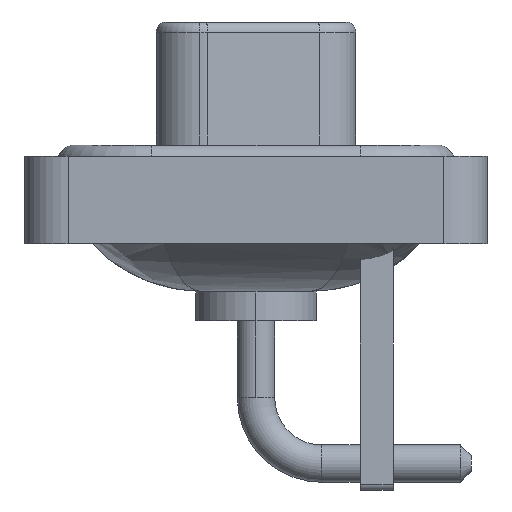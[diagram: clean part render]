
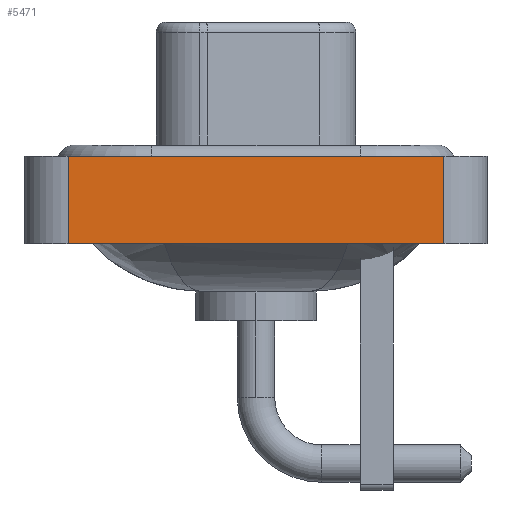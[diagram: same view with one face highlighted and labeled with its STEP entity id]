
A CAD part, left-side view. The second image highlights one B-rep face of the part: STEP entity #5471.
In plain terms, the highlighted planar face has unit normal (-1, 0, 0).
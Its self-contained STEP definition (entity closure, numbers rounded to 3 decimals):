
#958 = VERTEX_POINT ( 'NONE', #18567 ) ;
#1187 = CARTESIAN_POINT ( 'NONE',  ( -7.35, -8.55, 0.4 ) ) ;
#1277 = CARTESIAN_POINT ( 'NONE',  ( -7.35, -8.55, -3.6 ) ) ;
#1954 = CARTESIAN_POINT ( 'NONE',  ( -7.35, -8.55, -3.6 ) ) ;
#2816 = CARTESIAN_POINT ( 'NONE',  ( -7.35, -8.55, -3.6 ) ) ;
#2910 = DIRECTION ( 'NONE',  ( 0., 0., 1. ) ) ;
#4432 = VECTOR ( 'NONE', #15652, 1000. ) ;
#4685 = VECTOR ( 'NONE', #16803, 1000. ) ;
#4875 = EDGE_CURVE ( 'NONE', #958, #12931, #18037, .T. ) ;
#5471 = ADVANCED_FACE ( 'NONE', ( #10415 ), #8712, .T. ) ;
#5986 = ORIENTED_EDGE ( 'NONE', *, *, #4875, .F. ) ;
#6554 = CARTESIAN_POINT ( 'NONE',  ( -7.35, 8.55, 0.4 ) ) ;
#6995 = EDGE_CURVE ( 'NONE', #958, #9778, #15085, .T. ) ;
#7339 = LINE ( 'NONE', #11625, #9507 ) ;
#8279 = AXIS2_PLACEMENT_3D ( 'NONE', #2816, #11577, #2910 ) ;
#8712 = PLANE ( 'NONE',  #8279 ) ;
#9507 = VECTOR ( 'NONE', #13154, 1000. ) ;
#9778 = VERTEX_POINT ( 'NONE', #1277 ) ;
#10415 = FACE_OUTER_BOUND ( 'NONE', #10858, .T. ) ;
#10858 = EDGE_LOOP ( 'NONE', ( #15896, #11590, #5986, #11486 ) ) ;
#11139 = CARTESIAN_POINT ( 'NONE',  ( -7.35, -8.55, 0.4 ) ) ;
#11486 = ORIENTED_EDGE ( 'NONE', *, *, #6995, .T. ) ;
#11577 = DIRECTION ( 'NONE',  ( -1., 0., 0. ) ) ;
#11590 = ORIENTED_EDGE ( 'NONE', *, *, #18526, .F. ) ;
#11625 = CARTESIAN_POINT ( 'NONE',  ( -7.35, -8.55, -3.6 ) ) ;
#12048 = DIRECTION ( 'NONE',  ( 0., 0., 1. ) ) ;
#12931 = VERTEX_POINT ( 'NONE', #6554 ) ;
#13154 = DIRECTION ( 'NONE',  ( 0., 0., 1. ) ) ;
#13719 = EDGE_CURVE ( 'NONE', #9778, #16775, #7339, .T. ) ;
#15085 = LINE ( 'NONE', #1954, #4685 ) ;
#15652 = DIRECTION ( 'NONE',  ( 0., -1., 0. ) ) ;
#15896 = ORIENTED_EDGE ( 'NONE', *, *, #13719, .T. ) ;
#16775 = VERTEX_POINT ( 'NONE', #11139 ) ;
#16803 = DIRECTION ( 'NONE',  ( 0., -1., 0. ) ) ;
#17250 = VECTOR ( 'NONE', #12048, 1000. ) ;
#17948 = CARTESIAN_POINT ( 'NONE',  ( -7.35, 8.55, -3.6 ) ) ;
#18037 = LINE ( 'NONE', #17948, #17250 ) ;
#18526 = EDGE_CURVE ( 'NONE', #12931, #16775, #18704, .T. ) ;
#18567 = CARTESIAN_POINT ( 'NONE',  ( -7.35, 8.55, -3.6 ) ) ;
#18704 = LINE ( 'NONE', #1187, #4432 ) ;
